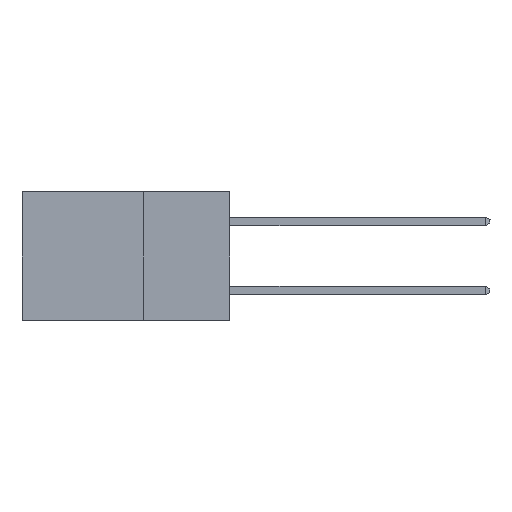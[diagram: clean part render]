
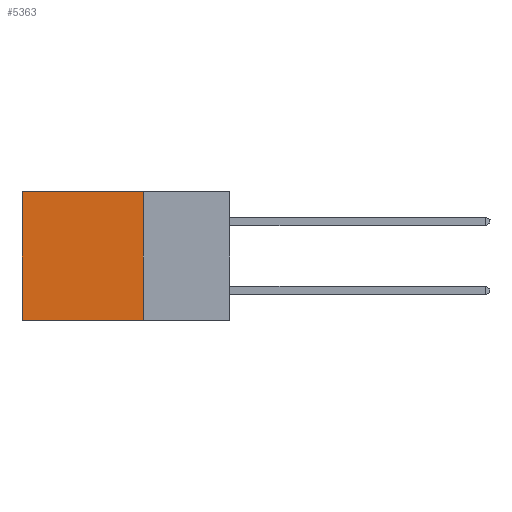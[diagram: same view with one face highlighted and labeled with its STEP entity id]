
A CAD part, left-side view. The second image highlights one B-rep face of the part: STEP entity #5363.
In plain terms, the highlighted planar face has unit normal (-1, 0, 0).
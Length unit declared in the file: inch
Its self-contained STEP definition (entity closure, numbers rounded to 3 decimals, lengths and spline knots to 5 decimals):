
#1890 = CARTESIAN_POINT ( 'NONE',  ( 0.2615, 0.6, -0.37 ) ) ;
#2246 = EDGE_CURVE ( 'NONE', #3810, #10021, #4711, .T. ) ;
#2299 = DIRECTION ( 'NONE',  ( 0., 0., -1. ) ) ;
#2353 = VECTOR ( 'NONE', #2299, 39.37008 ) ;
#3355 = LINE ( 'NONE', #3632, #8331 ) ;
#3380 = ORIENTED_EDGE ( 'NONE', *, *, #17186, .F. ) ;
#3632 = CARTESIAN_POINT ( 'NONE',  ( 0.2615, 0.25, -0.37 ) ) ;
#3810 = VERTEX_POINT ( 'NONE', #14123 ) ;
#4404 = EDGE_CURVE ( 'NONE', #6476, #10021, #14623, .T. ) ;
#4711 = LINE ( 'NONE', #4862, #6632 ) ;
#4862 = CARTESIAN_POINT ( 'NONE',  ( 0.2615, 0.25, -0.37 ) ) ;
#4981 = DIRECTION ( 'NONE',  ( 0., 1., 0. ) ) ;
#5363 = ADVANCED_FACE ( 'NONE', ( #17377 ), #25726, .F. ) ;
#5479 = AXIS2_PLACEMENT_3D ( 'NONE', #6985, #15346, #13284 ) ;
#6476 = VERTEX_POINT ( 'NONE', #12387 ) ;
#6632 = VECTOR ( 'NONE', #13070, 39.37008 ) ;
#6985 = CARTESIAN_POINT ( 'NONE',  ( 0.2615, 0.25, -0.37 ) ) ;
#8331 = VECTOR ( 'NONE', #17858, 39.37008 ) ;
#9656 = CARTESIAN_POINT ( 'NONE',  ( 0.2615, 0.6, -0.37 ) ) ;
#10021 = VERTEX_POINT ( 'NONE', #9656 ) ;
#12387 = CARTESIAN_POINT ( 'NONE',  ( 0.2615, 0.6, 0. ) ) ;
#12925 = LINE ( 'NONE', #15525, #19836 ) ;
#13070 = DIRECTION ( 'NONE',  ( 0., 1., 0. ) ) ;
#13284 = DIRECTION ( 'NONE',  ( 0., 0., -1. ) ) ;
#13424 = VERTEX_POINT ( 'NONE', #14726 ) ;
#14123 = CARTESIAN_POINT ( 'NONE',  ( 0.2615, 0.25, -0.37 ) ) ;
#14623 = LINE ( 'NONE', #1890, #2353 ) ;
#14726 = CARTESIAN_POINT ( 'NONE',  ( 0.2615, 0.25, 0. ) ) ;
#15346 = DIRECTION ( 'NONE',  ( 1., 0., 0. ) ) ;
#15525 = CARTESIAN_POINT ( 'NONE',  ( 0.2615, 0.25, 0. ) ) ;
#16840 = ORIENTED_EDGE ( 'NONE', *, *, #18929, .T. ) ;
#17186 = EDGE_CURVE ( 'NONE', #13424, #3810, #3355, .T. ) ;
#17377 = FACE_OUTER_BOUND ( 'NONE', #25939, .T. ) ;
#17858 = DIRECTION ( 'NONE',  ( 0., 0., -1. ) ) ;
#18929 = EDGE_CURVE ( 'NONE', #13424, #6476, #12925, .T. ) ;
#19643 = ORIENTED_EDGE ( 'NONE', *, *, #4404, .T. ) ;
#19836 = VECTOR ( 'NONE', #4981, 39.37008 ) ;
#19889 = ORIENTED_EDGE ( 'NONE', *, *, #2246, .F. ) ;
#25726 = PLANE ( 'NONE',  #5479 ) ;
#25939 = EDGE_LOOP ( 'NONE', ( #19643, #19889, #3380, #16840 ) ) ;
